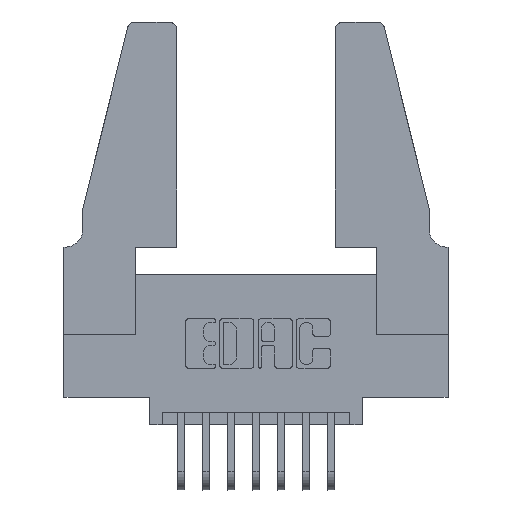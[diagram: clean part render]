
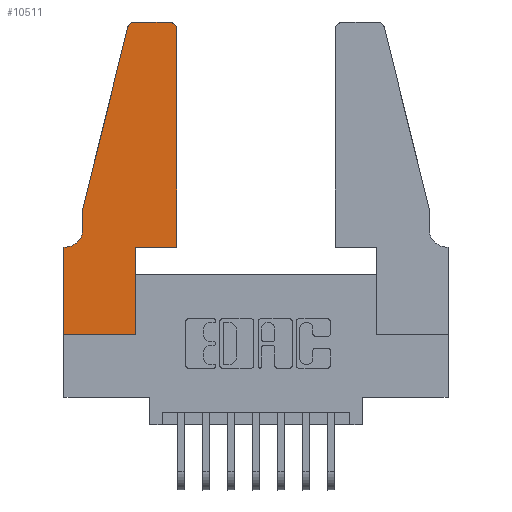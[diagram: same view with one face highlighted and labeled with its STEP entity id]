
A CAD part, top view. The second image highlights one B-rep face of the part: STEP entity #10511.
In plain terms, the highlighted planar face has unit normal (0, 0, 1).
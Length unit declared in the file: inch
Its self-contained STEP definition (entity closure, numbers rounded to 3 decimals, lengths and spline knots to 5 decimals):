
#62 = FACE_OUTER_BOUND ( 'NONE', #4152, .T. ) ;
#66 = DIRECTION ( 'NONE',  ( -1., 0., 0. ) ) ;
#161 = CARTESIAN_POINT ( 'NONE',  ( 0., 0., 0.37 ) ) ;
#205 = DIRECTION ( 'NONE',  ( -0.239, -0.971, 0. ) ) ;
#321 = CIRCLE ( 'NONE', #8114, 0.03 ) ;
#388 = EDGE_CURVE ( 'NONE', #13895, #11569, #8891, .T. ) ;
#812 = DIRECTION ( 'NONE',  ( -1., 0., 0. ) ) ;
#963 = DIRECTION ( 'NONE',  ( 0., 1., 0. ) ) ;
#968 = VERTEX_POINT ( 'NONE', #13950 ) ;
#995 = CARTESIAN_POINT ( 'NONE',  ( 0.4505, 1.22, 0.37 ) ) ;
#1016 = VERTEX_POINT ( 'NONE', #14170 ) ;
#1086 = EDGE_CURVE ( 'NONE', #7109, #11930, #7210, .T. ) ;
#1115 = DIRECTION ( 'NONE',  ( -1., 0., 0. ) ) ;
#1525 = EDGE_CURVE ( 'NONE', #3622, #4427, #11952, .T. ) ;
#1608 = DIRECTION ( 'NONE',  ( 1., 0., 0. ) ) ;
#1663 = EDGE_CURVE ( 'NONE', #11930, #7288, #321, .T. ) ;
#1902 = CARTESIAN_POINT ( 'NONE',  ( 0., 0., 0.37 ) ) ;
#2056 = CARTESIAN_POINT ( 'NONE',  ( 0.2865, 0.35, 0.37 ) ) ;
#2059 = LINE ( 'NONE', #2789, #7550 ) ;
#2243 = DIRECTION ( 'NONE',  ( 1., 0., 0. ) ) ;
#2381 = VECTOR ( 'NONE', #13965, 39.37008 ) ;
#2441 = CARTESIAN_POINT ( 'NONE',  ( 0.25487, 1.22718, 0.37 ) ) ;
#2772 = LINE ( 'NONE', #7516, #3625 ) ;
#2789 = CARTESIAN_POINT ( 'NONE',  ( 0., 0., 0.37 ) ) ;
#2825 = VECTOR ( 'NONE', #812, 39.37008 ) ;
#3160 = LINE ( 'NONE', #4153, #2825 ) ;
#3249 = AXIS2_PLACEMENT_3D ( 'NONE', #6433, #5303, #1115 ) ;
#3344 = CARTESIAN_POINT ( 'NONE',  ( 0.284, 1.22, 0.37 ) ) ;
#3349 = DIRECTION ( 'NONE',  ( 0., 0., 1. ) ) ;
#3469 = EDGE_CURVE ( 'NONE', #12423, #7109, #8544, .T. ) ;
#3481 = ORIENTED_EDGE ( 'NONE', *, *, #388, .T. ) ;
#3570 = CARTESIAN_POINT ( 'NONE',  ( 0., 0.35, 0.37 ) ) ;
#3617 = ORIENTED_EDGE ( 'NONE', *, *, #7344, .T. ) ;
#3622 = VERTEX_POINT ( 'NONE', #4826 ) ;
#3625 = VECTOR ( 'NONE', #963, 39.37008 ) ;
#3847 = VECTOR ( 'NONE', #6984, 39.37008 ) ;
#4152 = EDGE_LOOP ( 'NONE', ( #12965, #9985, #13445, #3617, #9699, #8307, #12087, #6596, #3481, #11257, #12715, #6073 ) ) ;
#4153 = CARTESIAN_POINT ( 'NONE',  ( 0.0755, 0.35, 0.37 ) ) ;
#4227 = CARTESIAN_POINT ( 'NONE',  ( 0.2865, 0.35, 0.37 ) ) ;
#4276 = CARTESIAN_POINT ( 'NONE',  ( 0.4205, 1.25, 0.37 ) ) ;
#4427 = VERTEX_POINT ( 'NONE', #12466 ) ;
#4826 = CARTESIAN_POINT ( 'NONE',  ( 0.0755, 0.42, 0.37 ) ) ;
#4853 = CARTESIAN_POINT ( 'NONE',  ( 0.284, 1.25, 0.37 ) ) ;
#5303 = DIRECTION ( 'NONE',  ( 0., 0., -1. ) ) ;
#5690 = DIRECTION ( 'NONE',  ( 1., 0., 0. ) ) ;
#5758 = CARTESIAN_POINT ( 'NONE',  ( 0.0755, 0.5, 0.37 ) ) ;
#5797 = DIRECTION ( 'NONE',  ( 0., 0., 1. ) ) ;
#6073 = ORIENTED_EDGE ( 'NONE', *, *, #3469, .T. ) ;
#6433 = CARTESIAN_POINT ( 'NONE',  ( 0.0055, 0.42, 0.37 ) ) ;
#6596 = ORIENTED_EDGE ( 'NONE', *, *, #12215, .T. ) ;
#6719 = CARTESIAN_POINT ( 'NONE',  ( 0.4205, 1.22, 0.37 ) ) ;
#6748 = EDGE_CURVE ( 'NONE', #4427, #968, #3160, .T. ) ;
#6767 = CARTESIAN_POINT ( 'NONE',  ( 0.4505, 0.35, 0.37 ) ) ;
#6806 = DIRECTION ( 'NONE',  ( 1., 0., 0. ) ) ;
#6817 = DIRECTION ( 'NONE',  ( 1., 0., 0. ) ) ;
#6984 = DIRECTION ( 'NONE',  ( 0., -1., 0. ) ) ;
#7109 = VERTEX_POINT ( 'NONE', #4276 ) ;
#7210 = LINE ( 'NONE', #13167, #9735 ) ;
#7288 = VERTEX_POINT ( 'NONE', #2441 ) ;
#7344 = EDGE_CURVE ( 'NONE', #1016, #3622, #8966, .T. ) ;
#7516 = CARTESIAN_POINT ( 'NONE',  ( 0.4505, 0.35, 0.37 ) ) ;
#7550 = VECTOR ( 'NONE', #1608, 39.37008 ) ;
#7918 = EDGE_CURVE ( 'NONE', #7288, #1016, #8428, .T. ) ;
#7941 = AXIS2_PLACEMENT_3D ( 'NONE', #6719, #3349, #2243 ) ;
#8017 = CARTESIAN_POINT ( 'NONE',  ( 0.2865, 0., 0.37 ) ) ;
#8114 = AXIS2_PLACEMENT_3D ( 'NONE', #3344, #12239, #6806 ) ;
#8145 = VERTEX_POINT ( 'NONE', #8582 ) ;
#8307 = ORIENTED_EDGE ( 'NONE', *, *, #6748, .T. ) ;
#8428 = LINE ( 'NONE', #5758, #13909 ) ;
#8544 = CIRCLE ( 'NONE', #7941, 0.03 ) ;
#8582 = CARTESIAN_POINT ( 'NONE',  ( 0.4505, 0.35, 0.37 ) ) ;
#8757 = EDGE_CURVE ( 'NONE', #968, #9400, #11749, .T. ) ;
#8832 = VECTOR ( 'NONE', #12435, 39.37008 ) ;
#8891 = LINE ( 'NONE', #2056, #2381 ) ;
#8966 = LINE ( 'NONE', #13454, #3847 ) ;
#8997 = EDGE_CURVE ( 'NONE', #11569, #8145, #10375, .T. ) ;
#9400 = VERTEX_POINT ( 'NONE', #1902 ) ;
#9699 = ORIENTED_EDGE ( 'NONE', *, *, #1525, .T. ) ;
#9735 = VECTOR ( 'NONE', #66, 39.37008 ) ;
#9985 = ORIENTED_EDGE ( 'NONE', *, *, #1663, .T. ) ;
#10375 = LINE ( 'NONE', #6767, #11570 ) ;
#10511 = ADVANCED_FACE ( 'NONE', ( #62 ), #11168, .T. ) ;
#11168 = PLANE ( 'NONE',  #12694 ) ;
#11257 = ORIENTED_EDGE ( 'NONE', *, *, #8997, .T. ) ;
#11365 = EDGE_CURVE ( 'NONE', #8145, #12423, #2772, .T. ) ;
#11569 = VERTEX_POINT ( 'NONE', #4227 ) ;
#11570 = VECTOR ( 'NONE', #6817, 39.37008 ) ;
#11749 = LINE ( 'NONE', #161, #8832 ) ;
#11930 = VERTEX_POINT ( 'NONE', #4853 ) ;
#11952 = CIRCLE ( 'NONE', #3249, 0.07 ) ;
#12087 = ORIENTED_EDGE ( 'NONE', *, *, #8757, .T. ) ;
#12215 = EDGE_CURVE ( 'NONE', #9400, #13895, #2059, .T. ) ;
#12239 = DIRECTION ( 'NONE',  ( 0., 0., 1. ) ) ;
#12423 = VERTEX_POINT ( 'NONE', #995 ) ;
#12435 = DIRECTION ( 'NONE',  ( 0., -1., 0. ) ) ;
#12466 = CARTESIAN_POINT ( 'NONE',  ( 0.0055, 0.35, 0.37 ) ) ;
#12694 = AXIS2_PLACEMENT_3D ( 'NONE', #3570, #5797, #5690 ) ;
#12715 = ORIENTED_EDGE ( 'NONE', *, *, #11365, .T. ) ;
#12965 = ORIENTED_EDGE ( 'NONE', *, *, #1086, .T. ) ;
#13167 = CARTESIAN_POINT ( 'NONE',  ( 0.2605, 1.25, 0.37 ) ) ;
#13445 = ORIENTED_EDGE ( 'NONE', *, *, #7918, .T. ) ;
#13454 = CARTESIAN_POINT ( 'NONE',  ( 0.0755, 0.5, 0.37 ) ) ;
#13895 = VERTEX_POINT ( 'NONE', #8017 ) ;
#13909 = VECTOR ( 'NONE', #205, 39.37008 ) ;
#13950 = CARTESIAN_POINT ( 'NONE',  ( 0., 0.35, 0.37 ) ) ;
#13965 = DIRECTION ( 'NONE',  ( 0., 1., 0. ) ) ;
#14170 = CARTESIAN_POINT ( 'NONE',  ( 0.0755, 0.5, 0.37 ) ) ;
